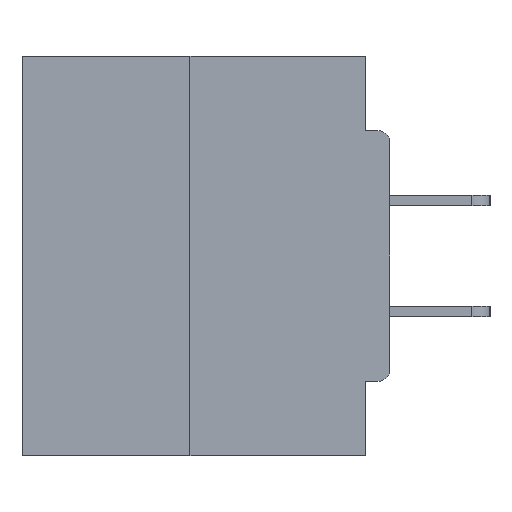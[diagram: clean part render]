
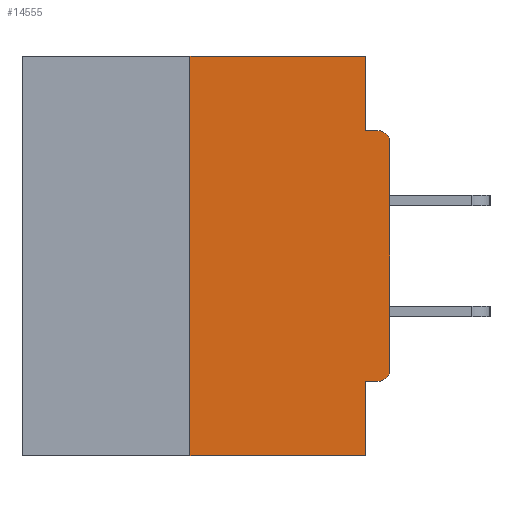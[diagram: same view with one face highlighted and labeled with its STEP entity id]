
A CAD part, left-side view. The second image highlights one B-rep face of the part: STEP entity #14555.
In plain terms, the highlighted planar face has unit normal (-1, 0, 0).
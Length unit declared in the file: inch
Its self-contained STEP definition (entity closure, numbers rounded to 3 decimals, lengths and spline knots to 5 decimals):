
#152 = VECTOR ( 'NONE', #15834, 39.37008 ) ;
#215 = LINE ( 'NONE', #10157, #22980 ) ;
#986 = LINE ( 'NONE', #21078, #10539 ) ;
#1311 = VECTOR ( 'NONE', #2626, 39.37008 ) ;
#2185 = ORIENTED_EDGE ( 'NONE', *, *, #11810, .F. ) ;
#2279 = EDGE_CURVE ( 'NONE', #24064, #27240, #10589, .T. ) ;
#2556 = EDGE_CURVE ( 'NONE', #24064, #14314, #14190, .T. ) ;
#2626 = DIRECTION ( 'NONE',  ( 0., 0., 1. ) ) ;
#2769 = EDGE_LOOP ( 'NONE', ( #19633, #31194, #14970, #14098, #27076, #13422, #19926, #17808, #2185, #5698 ) ) ;
#3042 = CARTESIAN_POINT ( 'NONE',  ( 0., 0.031, -0.4065 ) ) ;
#3112 = CARTESIAN_POINT ( 'NONE',  ( 0., 0.015, -0.4065 ) ) ;
#3335 = EDGE_CURVE ( 'NONE', #23258, #20360, #4862, .T. ) ;
#3698 = CARTESIAN_POINT ( 'NONE',  ( 0., 0.46, 0. ) ) ;
#3872 = DIRECTION ( 'NONE',  ( 1., 0., 0. ) ) ;
#4862 = CIRCLE ( 'NONE', #10046, 0.015 ) ;
#5698 = ORIENTED_EDGE ( 'NONE', *, *, #31551, .F. ) ;
#6276 = VERTEX_POINT ( 'NONE', #23185 ) ;
#6431 = CARTESIAN_POINT ( 'NONE',  ( 0., 0.46, -0.5 ) ) ;
#6855 = EDGE_CURVE ( 'NONE', #18075, #14957, #13906, .T. ) ;
#7165 = CARTESIAN_POINT ( 'NONE',  ( 0., 0., -0.1085 ) ) ;
#7360 = VECTOR ( 'NONE', #11129, 39.37008 ) ;
#8473 = CARTESIAN_POINT ( 'NONE',  ( 0., 0.015, -0.3915 ) ) ;
#8909 = DIRECTION ( 'NONE',  ( 0., 0., -1. ) ) ;
#8924 = CARTESIAN_POINT ( 'NONE',  ( 0., 0.25, -0.5 ) ) ;
#9717 = CARTESIAN_POINT ( 'NONE',  ( 0., 0.031, -0.0935 ) ) ;
#10046 = AXIS2_PLACEMENT_3D ( 'NONE', #12144, #27212, #22161 ) ;
#10084 = VECTOR ( 'NONE', #22277, 39.37008 ) ;
#10157 = CARTESIAN_POINT ( 'NONE',  ( 0., 0.46, 0. ) ) ;
#10285 = CARTESIAN_POINT ( 'NONE',  ( 0., 0.031, -0.5 ) ) ;
#10519 = AXIS2_PLACEMENT_3D ( 'NONE', #3698, #3872, #8909 ) ;
#10539 = VECTOR ( 'NONE', #18946, 39.37008 ) ;
#10589 = LINE ( 'NONE', #13048, #152 ) ;
#11129 = DIRECTION ( 'NONE',  ( 0., -1., 0. ) ) ;
#11348 = EDGE_CURVE ( 'NONE', #18075, #6276, #27578, .T. ) ;
#11564 = DIRECTION ( 'NONE',  ( -1., 0., 0. ) ) ;
#11683 = PLANE ( 'NONE',  #10519 ) ;
#11810 = EDGE_CURVE ( 'NONE', #20947, #20360, #25086, .T. ) ;
#12144 = CARTESIAN_POINT ( 'NONE',  ( 0., 0.015, -0.1085 ) ) ;
#12329 = CARTESIAN_POINT ( 'NONE',  ( 0., 0.25, 0. ) ) ;
#12415 = LINE ( 'NONE', #10285, #10084 ) ;
#13048 = CARTESIAN_POINT ( 'NONE',  ( 0., 0., -0.4065 ) ) ;
#13422 = ORIENTED_EDGE ( 'NONE', *, *, #2556, .T. ) ;
#13906 = LINE ( 'NONE', #6431, #7360 ) ;
#13991 = VERTEX_POINT ( 'NONE', #29991 ) ;
#14098 = ORIENTED_EDGE ( 'NONE', *, *, #17445, .F. ) ;
#14190 = CIRCLE ( 'NONE', #16840, 0.015 ) ;
#14314 = VERTEX_POINT ( 'NONE', #17420 ) ;
#14555 = ADVANCED_FACE ( 'NONE', ( #24144 ), #11683, .F. ) ;
#14957 = VERTEX_POINT ( 'NONE', #30468 ) ;
#14970 = ORIENTED_EDGE ( 'NONE', *, *, #6855, .T. ) ;
#15139 = CARTESIAN_POINT ( 'NONE',  ( 0., 0.015, -0.0935 ) ) ;
#15834 = DIRECTION ( 'NONE',  ( 0., 1., 0. ) ) ;
#16628 = EDGE_CURVE ( 'NONE', #14314, #23258, #28120, .T. ) ;
#16840 = AXIS2_PLACEMENT_3D ( 'NONE', #8473, #11564, #21574 ) ;
#17395 = DIRECTION ( 'NONE',  ( 0., 0., 1. ) ) ;
#17420 = CARTESIAN_POINT ( 'NONE',  ( 0., 0., -0.3915 ) ) ;
#17445 = EDGE_CURVE ( 'NONE', #27240, #14957, #12415, .T. ) ;
#17808 = ORIENTED_EDGE ( 'NONE', *, *, #3335, .T. ) ;
#18075 = VERTEX_POINT ( 'NONE', #8924 ) ;
#18946 = DIRECTION ( 'NONE',  ( 0., 0., -1. ) ) ;
#19445 = VECTOR ( 'NONE', #19990, 39.37008 ) ;
#19520 = CARTESIAN_POINT ( 'NONE',  ( 0., 0., -0.0935 ) ) ;
#19633 = ORIENTED_EDGE ( 'NONE', *, *, #25185, .F. ) ;
#19926 = ORIENTED_EDGE ( 'NONE', *, *, #16628, .T. ) ;
#19990 = DIRECTION ( 'NONE',  ( 0., -1., 0. ) ) ;
#20133 = DIRECTION ( 'NONE',  ( 0., -1., 0. ) ) ;
#20360 = VERTEX_POINT ( 'NONE', #15139 ) ;
#20947 = VERTEX_POINT ( 'NONE', #9717 ) ;
#21078 = CARTESIAN_POINT ( 'NONE',  ( 0., 0.031, 0. ) ) ;
#21574 = DIRECTION ( 'NONE',  ( 0., 0., -1. ) ) ;
#22161 = DIRECTION ( 'NONE',  ( 0., 0., -1. ) ) ;
#22277 = DIRECTION ( 'NONE',  ( 0., 0., -1. ) ) ;
#22736 = CARTESIAN_POINT ( 'NONE',  ( 0., 0., 0. ) ) ;
#22980 = VECTOR ( 'NONE', #20133, 39.37008 ) ;
#23185 = CARTESIAN_POINT ( 'NONE',  ( 0., 0.25, 0. ) ) ;
#23258 = VERTEX_POINT ( 'NONE', #7165 ) ;
#24064 = VERTEX_POINT ( 'NONE', #3112 ) ;
#24144 = FACE_OUTER_BOUND ( 'NONE', #2769, .T. ) ;
#25086 = LINE ( 'NONE', #19520, #19445 ) ;
#25185 = EDGE_CURVE ( 'NONE', #6276, #13991, #215, .T. ) ;
#27076 = ORIENTED_EDGE ( 'NONE', *, *, #2279, .F. ) ;
#27212 = DIRECTION ( 'NONE',  ( -1., 0., 0. ) ) ;
#27240 = VERTEX_POINT ( 'NONE', #3042 ) ;
#27280 = VECTOR ( 'NONE', #17395, 39.37008 ) ;
#27578 = LINE ( 'NONE', #12329, #27280 ) ;
#28120 = LINE ( 'NONE', #22736, #1311 ) ;
#29991 = CARTESIAN_POINT ( 'NONE',  ( 0., 0.031, 0. ) ) ;
#30468 = CARTESIAN_POINT ( 'NONE',  ( 0., 0.031, -0.5 ) ) ;
#31194 = ORIENTED_EDGE ( 'NONE', *, *, #11348, .F. ) ;
#31551 = EDGE_CURVE ( 'NONE', #13991, #20947, #986, .T. ) ;
